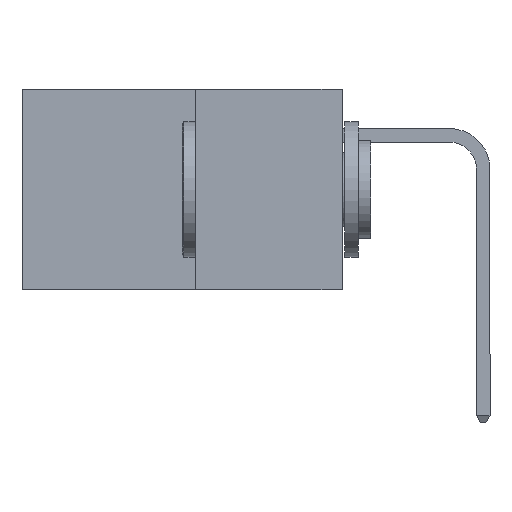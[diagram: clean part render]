
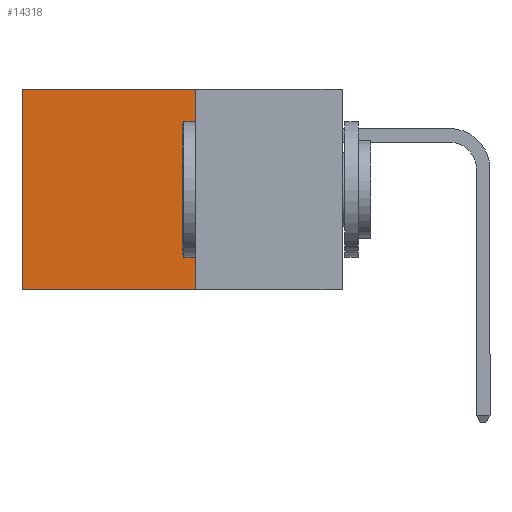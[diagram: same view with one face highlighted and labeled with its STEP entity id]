
A CAD part, left-side view. The second image highlights one B-rep face of the part: STEP entity #14318.
In plain terms, the highlighted planar face has unit normal (-1, 0, 0).
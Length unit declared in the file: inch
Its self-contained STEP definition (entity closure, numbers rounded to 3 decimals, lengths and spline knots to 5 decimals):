
#2174 = DIRECTION ( 'NONE',  ( 1., 0., 0. ) ) ;
#3150 = CARTESIAN_POINT ( 'NONE',  ( 0.277, 0.27, 0. ) ) ;
#3484 = DIRECTION ( 'NONE',  ( 0., 0., -1. ) ) ;
#4666 = DIRECTION ( 'NONE',  ( 0., 1., 0. ) ) ;
#4906 = VERTEX_POINT ( 'NONE', #14394 ) ;
#5058 = VECTOR ( 'NONE', #18227, 39.37008 ) ;
#5418 = CARTESIAN_POINT ( 'NONE',  ( 0.277, 0.59, 0. ) ) ;
#6422 = CARTESIAN_POINT ( 'NONE',  ( 0.277, 0.27, -0.37 ) ) ;
#6582 = CARTESIAN_POINT ( 'NONE',  ( 0.277, 0.59, -0.37 ) ) ;
#6900 = LINE ( 'NONE', #6422, #14218 ) ;
#8109 = CARTESIAN_POINT ( 'NONE',  ( 0.277, 0.27, -0.37 ) ) ;
#8517 = EDGE_CURVE ( 'NONE', #4906, #9732, #6900, .T. ) ;
#9573 = PLANE ( 'NONE',  #11044 ) ;
#9732 = VERTEX_POINT ( 'NONE', #15111 ) ;
#11044 = AXIS2_PLACEMENT_3D ( 'NONE', #8109, #2174, #12497 ) ;
#11176 = ORIENTED_EDGE ( 'NONE', *, *, #12787, .T. ) ;
#11334 = VERTEX_POINT ( 'NONE', #5418 ) ;
#11570 = LINE ( 'NONE', #3150, #18804 ) ;
#11747 = FACE_OUTER_BOUND ( 'NONE', #18984, .T. ) ;
#12056 = ORIENTED_EDGE ( 'NONE', *, *, #15941, .F. ) ;
#12148 = ORIENTED_EDGE ( 'NONE', *, *, #8517, .F. ) ;
#12497 = DIRECTION ( 'NONE',  ( 0., 0., -1. ) ) ;
#12787 = EDGE_CURVE ( 'NONE', #4906, #11334, #11570, .T. ) ;
#13041 = VECTOR ( 'NONE', #18048, 39.37008 ) ;
#13492 = LINE ( 'NONE', #13694, #13041 ) ;
#13694 = CARTESIAN_POINT ( 'NONE',  ( 0.277, 0.27, -0.37 ) ) ;
#14218 = VECTOR ( 'NONE', #3484, 39.37008 ) ;
#14318 = ADVANCED_FACE ( 'NONE', ( #11747 ), #9573, .F. ) ;
#14394 = CARTESIAN_POINT ( 'NONE',  ( 0.277, 0.27, 0. ) ) ;
#14929 = EDGE_CURVE ( 'NONE', #11334, #17114, #16740, .T. ) ;
#15017 = ORIENTED_EDGE ( 'NONE', *, *, #14929, .T. ) ;
#15111 = CARTESIAN_POINT ( 'NONE',  ( 0.277, 0.27, -0.37 ) ) ;
#15941 = EDGE_CURVE ( 'NONE', #9732, #17114, #13492, .T. ) ;
#16740 = LINE ( 'NONE', #6582, #5058 ) ;
#17114 = VERTEX_POINT ( 'NONE', #18071 ) ;
#18048 = DIRECTION ( 'NONE',  ( 0., 1., 0. ) ) ;
#18071 = CARTESIAN_POINT ( 'NONE',  ( 0.277, 0.59, -0.37 ) ) ;
#18227 = DIRECTION ( 'NONE',  ( 0., 0., -1. ) ) ;
#18804 = VECTOR ( 'NONE', #4666, 39.37008 ) ;
#18984 = EDGE_LOOP ( 'NONE', ( #15017, #12056, #12148, #11176 ) ) ;
